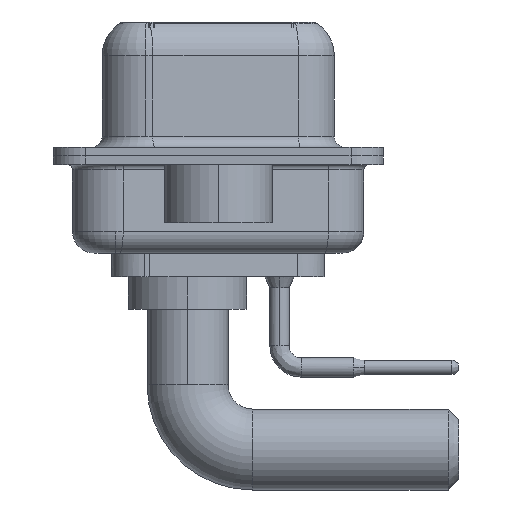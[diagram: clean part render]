
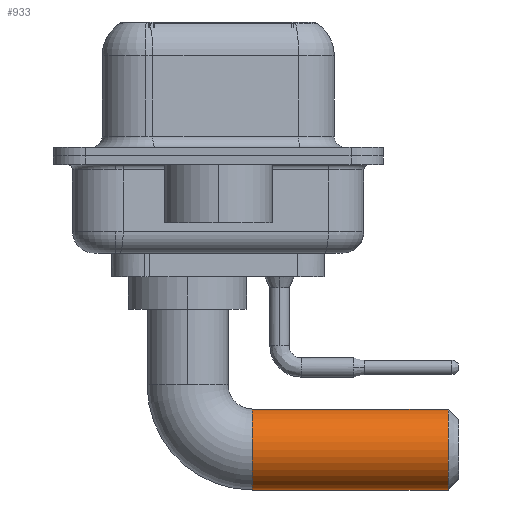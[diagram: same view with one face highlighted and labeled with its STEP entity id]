
A CAD part, left-side view. The second image highlights one B-rep face of the part: STEP entity #933.
In plain terms, the highlighted cylindrical face has radius 1.875 mm (diameter 3.75 mm), a partial arc.
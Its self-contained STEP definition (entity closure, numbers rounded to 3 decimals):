
#30 = LINE ( 'NONE', #939, #15955 ) ;
#108 = DIRECTION ( 'NONE',  ( 0., -1., 0. ) ) ;
#933 = ADVANCED_FACE ( 'NONE', ( #986 ), #4391, .T. ) ;
#939 = CARTESIAN_POINT ( 'NONE',  ( 0., -3., -8.375 ) ) ;
#986 = FACE_OUTER_BOUND ( 'NONE', #19297, .T. ) ;
#2183 = CARTESIAN_POINT ( 'NONE',  ( 0., -3., -4.625 ) ) ;
#2532 = DIRECTION ( 'NONE',  ( 0., -1., 0. ) ) ;
#3162 = CARTESIAN_POINT ( 'NONE',  ( 0., -12.07, -8.375 ) ) ;
#3524 = VERTEX_POINT ( 'NONE', #5353 ) ;
#3909 = VERTEX_POINT ( 'NONE', #10243 ) ;
#4327 = DIRECTION ( 'NONE',  ( -1., 0., 0. ) ) ;
#4391 = CYLINDRICAL_SURFACE ( 'NONE', #17086, 1.875 ) ;
#4858 = EDGE_CURVE ( 'NONE', #14207, #3524, #9660, .T. ) ;
#5353 = CARTESIAN_POINT ( 'NONE',  ( 0., -12.07, -4.625 ) ) ;
#8355 = VERTEX_POINT ( 'NONE', #16673 ) ;
#8360 = CARTESIAN_POINT ( 'NONE',  ( 0., -3., -6.5 ) ) ;
#8639 = ORIENTED_EDGE ( 'NONE', *, *, #12293, .T. ) ;
#9209 = DIRECTION ( 'NONE',  ( 0., 0., -1. ) ) ;
#9660 = CIRCLE ( 'NONE', #15144, 1.875 ) ;
#10243 = CARTESIAN_POINT ( 'NONE',  ( 0., -3., -8.375 ) ) ;
#10711 = EDGE_CURVE ( 'NONE', #8355, #3524, #15008, .T. ) ;
#12293 = EDGE_CURVE ( 'NONE', #8355, #3909, #19306, .T. ) ;
#12802 = VECTOR ( 'NONE', #13396, 1000. ) ;
#13396 = DIRECTION ( 'NONE',  ( 0., -1., 0. ) ) ;
#13399 = ORIENTED_EDGE ( 'NONE', *, *, #10711, .F. ) ;
#13812 = DIRECTION ( 'NONE',  ( 0., -1., 0. ) ) ;
#13898 = DIRECTION ( 'NONE',  ( 0., 0., -1. ) ) ;
#14025 = CARTESIAN_POINT ( 'NONE',  ( 0., -3., -6.5 ) ) ;
#14207 = VERTEX_POINT ( 'NONE', #3162 ) ;
#15008 = LINE ( 'NONE', #2183, #12802 ) ;
#15144 = AXIS2_PLACEMENT_3D ( 'NONE', #15302, #18738, #13898 ) ;
#15302 = CARTESIAN_POINT ( 'NONE',  ( 0., -12.07, -6.5 ) ) ;
#15955 = VECTOR ( 'NONE', #2532, 1000. ) ;
#16673 = CARTESIAN_POINT ( 'NONE',  ( 0., -3., -4.625 ) ) ;
#17086 = AXIS2_PLACEMENT_3D ( 'NONE', #14025, #13812, #9209 ) ;
#17564 = EDGE_CURVE ( 'NONE', #3909, #14207, #30, .T. ) ;
#18266 = ORIENTED_EDGE ( 'NONE', *, *, #17564, .T. ) ;
#18738 = DIRECTION ( 'NONE',  ( 0., 1., 0. ) ) ;
#19297 = EDGE_LOOP ( 'NONE', ( #13399, #8639, #18266, #19409 ) ) ;
#19306 = CIRCLE ( 'NONE', #20704, 1.875 ) ;
#19409 = ORIENTED_EDGE ( 'NONE', *, *, #4858, .T. ) ;
#20704 = AXIS2_PLACEMENT_3D ( 'NONE', #8360, #108, #4327 ) ;
